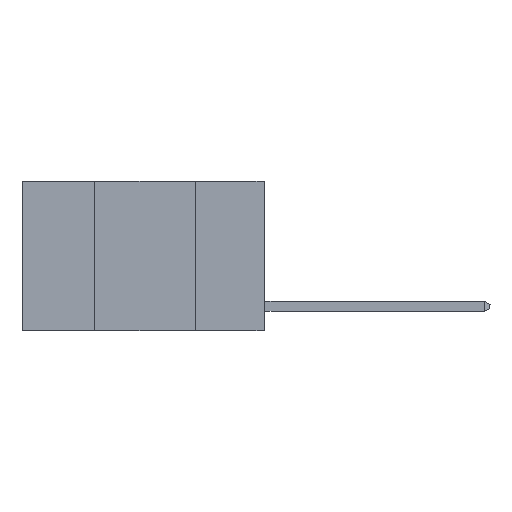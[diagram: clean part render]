
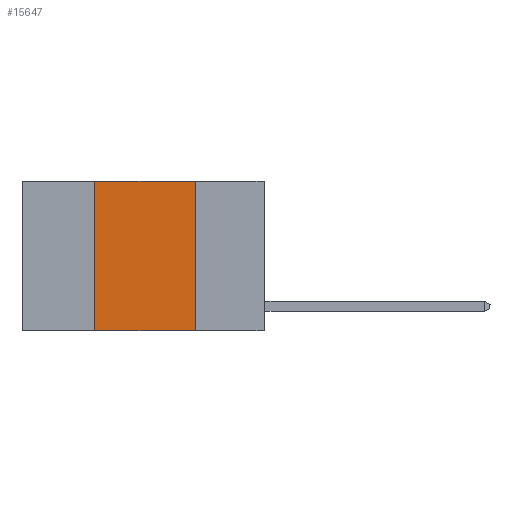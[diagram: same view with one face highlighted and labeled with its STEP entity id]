
A CAD part, left-side view. The second image highlights one B-rep face of the part: STEP entity #15647.
In plain terms, the highlighted planar face has unit normal (-1, 0, 0).
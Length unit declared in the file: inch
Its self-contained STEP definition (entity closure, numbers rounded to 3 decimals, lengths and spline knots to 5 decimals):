
#9 = VERTEX_POINT ( 'NONE', #24209 ) ;
#367 = ORIENTED_EDGE ( 'NONE', *, *, #10821, .F. ) ;
#1161 = CARTESIAN_POINT ( 'NONE',  ( 0., 0.6, 0. ) ) ;
#1573 = DIRECTION ( 'NONE',  ( 0., 0., 1. ) ) ;
#1713 = EDGE_CURVE ( 'NONE', #9, #8893, #18914, .T. ) ;
#2624 = EDGE_CURVE ( 'NONE', #9505, #9, #19172, .T. ) ;
#2853 = VERTEX_POINT ( 'NONE', #24501 ) ;
#4398 = AXIS2_PLACEMENT_3D ( 'NONE', #1161, #17865, #15911 ) ;
#5304 = CARTESIAN_POINT ( 'NONE',  ( 0., 0.42, -0.37 ) ) ;
#5442 = CARTESIAN_POINT ( 'NONE',  ( 0., 0.17, 0. ) ) ;
#6808 = CARTESIAN_POINT ( 'NONE',  ( 0., 0.6, 0. ) ) ;
#7776 = VECTOR ( 'NONE', #13109, 39.37008 ) ;
#8667 = VECTOR ( 'NONE', #15513, 39.37008 ) ;
#8893 = VERTEX_POINT ( 'NONE', #5442 ) ;
#9472 = VECTOR ( 'NONE', #24860, 39.37008 ) ;
#9505 = VERTEX_POINT ( 'NONE', #5304 ) ;
#9782 = FACE_OUTER_BOUND ( 'NONE', #17453, .T. ) ;
#10150 = ORIENTED_EDGE ( 'NONE', *, *, #2624, .F. ) ;
#10821 = EDGE_CURVE ( 'NONE', #8893, #2853, #11220, .T. ) ;
#11220 = LINE ( 'NONE', #19181, #7776 ) ;
#12025 = ORIENTED_EDGE ( 'NONE', *, *, #12106, .T. ) ;
#12106 = EDGE_CURVE ( 'NONE', #9505, #2853, #14660, .T. ) ;
#13109 = DIRECTION ( 'NONE',  ( 0., 0., -1. ) ) ;
#14660 = LINE ( 'NONE', #25944, #8667 ) ;
#15513 = DIRECTION ( 'NONE',  ( 0., -1., 0. ) ) ;
#15647 = ADVANCED_FACE ( 'NONE', ( #9782 ), #23562, .F. ) ;
#15911 = DIRECTION ( 'NONE',  ( 0., 0., -1. ) ) ;
#17453 = EDGE_LOOP ( 'NONE', ( #367, #19762, #10150, #12025 ) ) ;
#17865 = DIRECTION ( 'NONE',  ( 1., 0., 0. ) ) ;
#18914 = LINE ( 'NONE', #6808, #9472 ) ;
#19172 = LINE ( 'NONE', #21873, #19506 ) ;
#19181 = CARTESIAN_POINT ( 'NONE',  ( 0., 0.17, 0. ) ) ;
#19506 = VECTOR ( 'NONE', #1573, 39.37008 ) ;
#19762 = ORIENTED_EDGE ( 'NONE', *, *, #1713, .F. ) ;
#21873 = CARTESIAN_POINT ( 'NONE',  ( 0., 0.42, 0. ) ) ;
#23562 = PLANE ( 'NONE',  #4398 ) ;
#24209 = CARTESIAN_POINT ( 'NONE',  ( 0., 0.42, 0. ) ) ;
#24501 = CARTESIAN_POINT ( 'NONE',  ( 0., 0.17, -0.37 ) ) ;
#24860 = DIRECTION ( 'NONE',  ( 0., -1., 0. ) ) ;
#25944 = CARTESIAN_POINT ( 'NONE',  ( 0., 0.6, -0.37 ) ) ;
